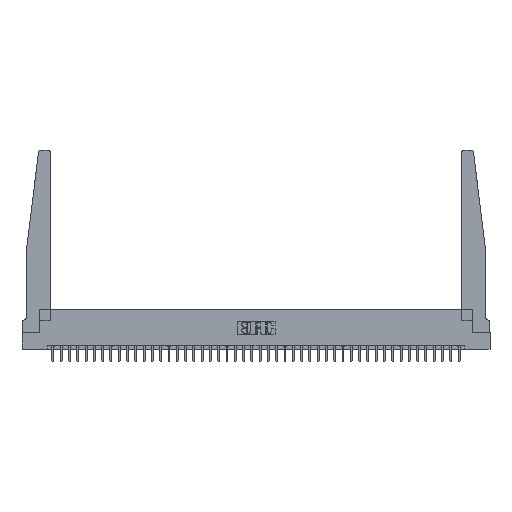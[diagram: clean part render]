
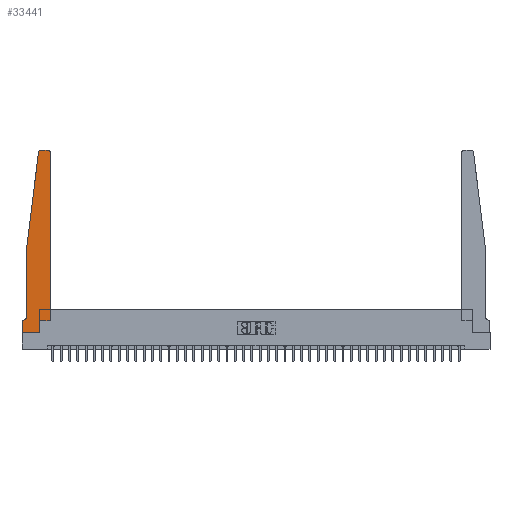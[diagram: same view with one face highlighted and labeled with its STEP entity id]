
A CAD part, top view. The second image highlights one B-rep face of the part: STEP entity #33441.
In plain terms, the highlighted planar face has unit normal (0, 0, 1).
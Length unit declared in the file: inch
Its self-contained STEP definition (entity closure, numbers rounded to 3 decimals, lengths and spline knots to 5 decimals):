
#34 = CARTESIAN_POINT ( 'NONE',  ( 0.2605, 0.18, 0.37 ) ) ;
#246 = LINE ( 'NONE', #31781, #21851 ) ;
#271 = CARTESIAN_POINT ( 'NONE',  ( 0., 0., 0.37 ) ) ;
#1372 = CARTESIAN_POINT ( 'NONE',  ( 0.25, 2.75, 0.37 ) ) ;
#1649 = ORIENTED_EDGE ( 'NONE', *, *, #29139, .T. ) ;
#1678 = VECTOR ( 'NONE', #16498, 39.37008 ) ;
#2047 = CARTESIAN_POINT ( 'NONE',  ( 0., 0.1875, 0.37 ) ) ;
#2438 = VERTEX_POINT ( 'NONE', #14341 ) ;
#2654 = DIRECTION ( 'NONE',  ( 0., -1., 0. ) ) ;
#2867 = CARTESIAN_POINT ( 'NONE',  ( 0.2605, 0., 0.37 ) ) ;
#3202 = VECTOR ( 'NONE', #35182, 39.37008 ) ;
#3210 = VERTEX_POINT ( 'NONE', #28315 ) ;
#3247 = EDGE_CURVE ( 'NONE', #3210, #2438, #7186, .T. ) ;
#3942 = CIRCLE ( 'NONE', #10200, 0.03 ) ;
#4185 = CARTESIAN_POINT ( 'NONE',  ( 0.2605, 0.18, 0.37 ) ) ;
#5473 = ORIENTED_EDGE ( 'NONE', *, *, #22176, .T. ) ;
#6307 = DIRECTION ( 'NONE',  ( 0., 1., 0. ) ) ;
#7107 = DIRECTION ( 'NONE',  ( 0., 0., 1. ) ) ;
#7142 = ORIENTED_EDGE ( 'NONE', *, *, #9862, .T. ) ;
#7186 = LINE ( 'NONE', #31324, #35799 ) ;
#7403 = LINE ( 'NONE', #13658, #1678 ) ;
#7497 = CARTESIAN_POINT ( 'NONE',  ( 0.065, 0.1875, 0.37 ) ) ;
#8316 = EDGE_CURVE ( 'NONE', #21604, #13249, #12429, .T. ) ;
#8890 = DIRECTION ( 'NONE',  ( 0., 0., -1. ) ) ;
#9719 = ORIENTED_EDGE ( 'NONE', *, *, #12493, .T. ) ;
#9862 = EDGE_CURVE ( 'NONE', #2438, #23652, #3942, .T. ) ;
#9998 = VERTEX_POINT ( 'NONE', #28452 ) ;
#10200 = AXIS2_PLACEMENT_3D ( 'NONE', #23944, #7107, #15172 ) ;
#10228 = CARTESIAN_POINT ( 'NONE',  ( 0.065, 1.25, 0.37 ) ) ;
#10507 = ORIENTED_EDGE ( 'NONE', *, *, #32440, .T. ) ;
#10950 = CARTESIAN_POINT ( 'NONE',  ( 0.395, 2.75, 0.37 ) ) ;
#11462 = CARTESIAN_POINT ( 'NONE',  ( 0.27653, 2.72, 0.37 ) ) ;
#11829 = EDGE_LOOP ( 'NONE', ( #31573, #10507, #13101, #31812, #25109, #16985, #5473, #9719, #1649, #36181, #15888, #7142 ) ) ;
#12429 = LINE ( 'NONE', #7497, #25122 ) ;
#12493 = EDGE_CURVE ( 'NONE', #9998, #34302, #30250, .T. ) ;
#13101 = ORIENTED_EDGE ( 'NONE', *, *, #35295, .T. ) ;
#13249 = VERTEX_POINT ( 'NONE', #2047 ) ;
#13278 = VERTEX_POINT ( 'NONE', #34 ) ;
#13338 = CARTESIAN_POINT ( 'NONE',  ( 0.065, 0.2375, 0.37 ) ) ;
#13506 = VERTEX_POINT ( 'NONE', #13338 ) ;
#13658 = CARTESIAN_POINT ( 'NONE',  ( 0.425, 0.18, 0.37 ) ) ;
#14341 = CARTESIAN_POINT ( 'NONE',  ( 0.425, 2.72, 0.37 ) ) ;
#15172 = DIRECTION ( 'NONE',  ( 1., 0., 0. ) ) ;
#15284 = DIRECTION ( 'NONE',  ( 0., 0., 1. ) ) ;
#15888 = ORIENTED_EDGE ( 'NONE', *, *, #3247, .T. ) ;
#16232 = CARTESIAN_POINT ( 'NONE',  ( 0., 0.1875, 0.37 ) ) ;
#16498 = DIRECTION ( 'NONE',  ( 1., 0., 0. ) ) ;
#16985 = ORIENTED_EDGE ( 'NONE', *, *, #8316, .T. ) ;
#17564 = VECTOR ( 'NONE', #27259, 39.37008 ) ;
#17724 = DIRECTION ( 'NONE',  ( 1., 0., 0. ) ) ;
#17747 = DIRECTION ( 'NONE',  ( 0., -1., 0. ) ) ;
#18867 = DIRECTION ( 'NONE',  ( 1., 0., 0. ) ) ;
#19281 = DIRECTION ( 'NONE',  ( 0., 0., 1. ) ) ;
#19760 = CIRCLE ( 'NONE', #27244, 0.03 ) ;
#19989 = DIRECTION ( 'NONE',  ( -1., 0., 0. ) ) ;
#20217 = VECTOR ( 'NONE', #24078, 39.37008 ) ;
#20790 = CARTESIAN_POINT ( 'NONE',  ( 0.065, 1.25, 0.37 ) ) ;
#21448 = VECTOR ( 'NONE', #18867, 39.37008 ) ;
#21593 = EDGE_CURVE ( 'NONE', #13506, #21604, #29058, .T. ) ;
#21604 = VERTEX_POINT ( 'NONE', #22660 ) ;
#21851 = VECTOR ( 'NONE', #17747, 39.37008 ) ;
#21960 = DIRECTION ( 'NONE',  ( 1., 0., 0. ) ) ;
#22176 = EDGE_CURVE ( 'NONE', #13249, #9998, #23284, .T. ) ;
#22660 = CARTESIAN_POINT ( 'NONE',  ( 0.015, 0.1875, 0.37 ) ) ;
#23234 = LINE ( 'NONE', #4185, #20217 ) ;
#23284 = LINE ( 'NONE', #271, #25911 ) ;
#23550 = VERTEX_POINT ( 'NONE', #31750 ) ;
#23652 = VERTEX_POINT ( 'NONE', #10950 ) ;
#23813 = EDGE_CURVE ( 'NONE', #13278, #3210, #7403, .T. ) ;
#23944 = CARTESIAN_POINT ( 'NONE',  ( 0.395, 2.72, 0.37 ) ) ;
#24078 = DIRECTION ( 'NONE',  ( 0., 1., 0. ) ) ;
#25109 = ORIENTED_EDGE ( 'NONE', *, *, #21593, .T. ) ;
#25122 = VECTOR ( 'NONE', #35687, 39.37008 ) ;
#25911 = VECTOR ( 'NONE', #2654, 39.37008 ) ;
#27244 = AXIS2_PLACEMENT_3D ( 'NONE', #11462, #15284, #17724 ) ;
#27259 = DIRECTION ( 'NONE',  ( -1., 0., 0. ) ) ;
#28315 = CARTESIAN_POINT ( 'NONE',  ( 0.425, 0.18, 0.37 ) ) ;
#28452 = CARTESIAN_POINT ( 'NONE',  ( 0., 0., 0.37 ) ) ;
#29058 = CIRCLE ( 'NONE', #32055, 0.05 ) ;
#29139 = EDGE_CURVE ( 'NONE', #34302, #13278, #23234, .T. ) ;
#29156 = LINE ( 'NONE', #20790, #3202 ) ;
#30250 = LINE ( 'NONE', #35699, #21448 ) ;
#30756 = CARTESIAN_POINT ( 'NONE',  ( 0.24675, 2.72367, 0.37 ) ) ;
#31324 = CARTESIAN_POINT ( 'NONE',  ( 0.425, 0.18, 0.37 ) ) ;
#31557 = AXIS2_PLACEMENT_3D ( 'NONE', #16232, #19281, #21960 ) ;
#31573 = ORIENTED_EDGE ( 'NONE', *, *, #32157, .T. ) ;
#31750 = CARTESIAN_POINT ( 'NONE',  ( 0.27653, 2.75, 0.37 ) ) ;
#31769 = CARTESIAN_POINT ( 'NONE',  ( 0.015, 0.2375, 0.37 ) ) ;
#31781 = CARTESIAN_POINT ( 'NONE',  ( 0.065, 1.25, 0.37 ) ) ;
#31812 = ORIENTED_EDGE ( 'NONE', *, *, #33754, .T. ) ;
#32055 = AXIS2_PLACEMENT_3D ( 'NONE', #31769, #8890, #19989 ) ;
#32157 = EDGE_CURVE ( 'NONE', #23652, #23550, #35175, .T. ) ;
#32440 = EDGE_CURVE ( 'NONE', #23550, #35064, #19760, .T. ) ;
#32690 = VERTEX_POINT ( 'NONE', #10228 ) ;
#33018 = PLANE ( 'NONE',  #31557 ) ;
#33317 = FACE_OUTER_BOUND ( 'NONE', #11829, .T. ) ;
#33441 = ADVANCED_FACE ( 'NONE', ( #33317 ), #33018, .T. ) ;
#33754 = EDGE_CURVE ( 'NONE', #32690, #13506, #246, .T. ) ;
#34302 = VERTEX_POINT ( 'NONE', #2867 ) ;
#35064 = VERTEX_POINT ( 'NONE', #30756 ) ;
#35175 = LINE ( 'NONE', #1372, #17564 ) ;
#35182 = DIRECTION ( 'NONE',  ( -0.122, -0.992, 0. ) ) ;
#35295 = EDGE_CURVE ( 'NONE', #35064, #32690, #29156, .T. ) ;
#35687 = DIRECTION ( 'NONE',  ( -1., 0., 0. ) ) ;
#35699 = CARTESIAN_POINT ( 'NONE',  ( 0., 0., 0.37 ) ) ;
#35799 = VECTOR ( 'NONE', #6307, 39.37008 ) ;
#36181 = ORIENTED_EDGE ( 'NONE', *, *, #23813, .T. ) ;
